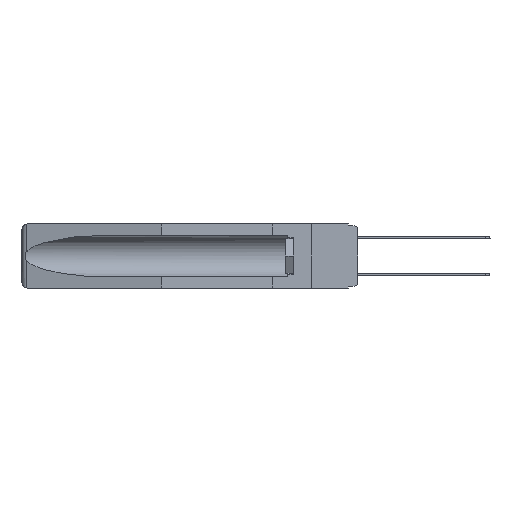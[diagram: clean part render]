
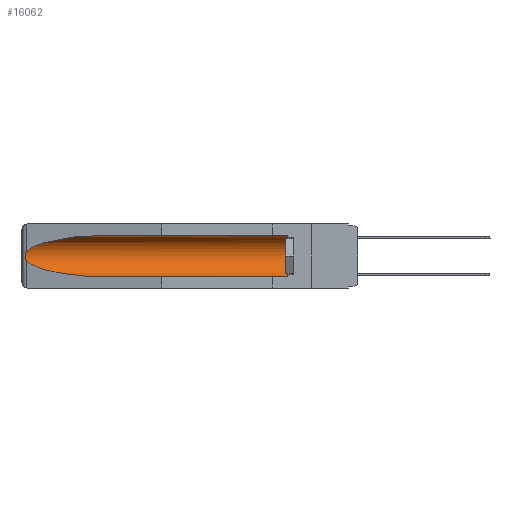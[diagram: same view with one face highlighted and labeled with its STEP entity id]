
A CAD part, left-side view. The second image highlights one B-rep face of the part: STEP entity #16062.
In plain terms, the highlighted cylindrical face has radius 2.857 mm (diameter 5.715 mm), a partial arc.
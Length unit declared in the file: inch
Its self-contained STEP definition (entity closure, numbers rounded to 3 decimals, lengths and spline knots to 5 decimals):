
#847 = CARTESIAN_POINT ( 'NONE',  ( 0.26537, 1.52718, -0.19328 ) ) ;
#1790 = EDGE_LOOP ( 'NONE', ( #23302, #11024, #22615, #20411, #14266, #4914 ) ) ;
#2506 = DIRECTION ( 'NONE',  ( 0., -1., 0. ) ) ;
#2961 = CARTESIAN_POINT ( 'NONE',  ( 0.26597, 1.5296, -0.19026 ) ) ;
#3761 = VERTEX_POINT ( 'NONE', #15420 ) ;
#3801 = AXIS2_PLACEMENT_3D ( 'NONE', #19124, #2506, #17112 ) ;
#4325 = EDGE_CURVE ( 'NONE', #20828, #23090, #21480, .T. ) ;
#4765 = CARTESIAN_POINT ( 'NONE',  ( 0.155, -0.30754, -0.059 ) ) ;
#4914 = ORIENTED_EDGE ( 'NONE', *, *, #7390, .T. ) ;
#5278 = CARTESIAN_POINT ( 'NONE',  ( 0.155, -0.30754, -0.284 ) ) ;
#5702 = EDGE_CURVE ( 'NONE', #15886, #20014, #6276, .T. ) ;
#6276 = B_SPLINE_CURVE_WITH_KNOTS ( 'NONE', 3,
 ( #13979, #10248, #6678, #15747, #21318, #15583, #19163, #23008, #2961, #847 ),
 .UNSPECIFIED., .F., .F.,
 ( 4, 2, 2, 2, 4 ),
 ( 0., 0.00029, 0.00058, 0.00087, 0.00117 ),
 .UNSPECIFIED. ) ;
#6293 = CARTESIAN_POINT ( 'NONE',  ( 0.25451, 1.48313, -0.24835 ) ) ;
#6678 = CARTESIAN_POINT ( 'NONE',  ( 0.26654, 1.53092, -0.15636 ) ) ;
#6847 = CARTESIAN_POINT ( 'NONE',  ( 0.155, 0.126, -0.059 ) ) ;
#7017 = CARTESIAN_POINT ( 'NONE',  ( 0.155, -0.30754, -0.1715 ) ) ;
#7390 = EDGE_CURVE ( 'NONE', #23090, #17053, #17417, .T. ) ;
#7773 = EDGE_CURVE ( 'NONE', #17053, #15886, #18972, .T. ) ;
#7809 = CYLINDRICAL_SURFACE ( 'NONE', #11198, 0.1125 ) ;
#8003 = CARTESIAN_POINT ( 'NONE',  ( 0.26537, 1.52718, -0.14972 ) ) ;
#8981 = CARTESIAN_POINT ( 'NONE',  ( 0.26537, 1.52718, -0.19328 ) ) ;
#9555 = CARTESIAN_POINT ( 'NONE',  ( 0.155, 1.07973, -0.059 ) ) ;
#10248 = CARTESIAN_POINT ( 'NONE',  ( 0.26597, 1.52961, -0.15275 ) ) ;
#11024 = ORIENTED_EDGE ( 'NONE', *, *, #5702, .T. ) ;
#11198 = AXIS2_PLACEMENT_3D ( 'NONE', #7017, #14158, #19795 ) ;
#11314 = CARTESIAN_POINT ( 'NONE',  ( 0.21114, 1.30732, -0.059 ) ) ;
#11334 = CARTESIAN_POINT ( 'NONE',  ( 0.155, 1.07973, -0.059 ) ) ;
#13169 = VECTOR ( 'NONE', #17492, 39.37008 ) ;
#13376 = CARTESIAN_POINT ( 'NONE',  ( 0.25451, 1.48313, -0.09465 ) ) ;
#13979 = CARTESIAN_POINT ( 'NONE',  ( 0.26537, 1.52718, -0.14972 ) ) ;
#14158 = DIRECTION ( 'NONE',  ( 0., 1., 0. ) ) ;
#14266 = ORIENTED_EDGE ( 'NONE', *, *, #4325, .T. ) ;
#14455 = EDGE_CURVE ( 'NONE', #20014, #3761, #14747, .T. ) ;
#14586 = VECTOR ( 'NONE', #19842, 39.37008 ) ;
#14747 =( BOUNDED_CURVE ( )  B_SPLINE_CURVE ( 3, ( #19119, #6293, #21102, #19189 ),
 .UNSPECIFIED., .F., .F. ) 
 B_SPLINE_CURVE_WITH_KNOTS ( ( 4, 4 ),
 ( 0.1948, 1.5708 ),
 .UNSPECIFIED. ) 
 CURVE ( )  GEOMETRIC_REPRESENTATION_ITEM ( )  RATIONAL_B_SPLINE_CURVE ( ( 1., 0.848, 0.848, 1. ) ) 
 REPRESENTATION_ITEM ( '' )  );
#15420 = CARTESIAN_POINT ( 'NONE',  ( 0.155, 1.07973, -0.284 ) ) ;
#15583 = CARTESIAN_POINT ( 'NONE',  ( 0.2675, 1.53308, -0.17534 ) ) ;
#15747 = CARTESIAN_POINT ( 'NONE',  ( 0.2673, 1.5327, -0.16383 ) ) ;
#15886 = VERTEX_POINT ( 'NONE', #19182 ) ;
#16062 = ADVANCED_FACE ( 'NONE', ( #20887 ), #7809, .F. ) ;
#16747 = EDGE_CURVE ( 'NONE', #20828, #3761, #19424, .T. ) ;
#17053 = VERTEX_POINT ( 'NONE', #11334 ) ;
#17112 = DIRECTION ( 'NONE',  ( 0., 0., 1. ) ) ;
#17417 = LINE ( 'NONE', #4765, #13169 ) ;
#17492 = DIRECTION ( 'NONE',  ( 0., 1., 0. ) ) ;
#18972 =( BOUNDED_CURVE ( )  B_SPLINE_CURVE ( 3, ( #9555, #11314, #13376, #8003 ),
 .UNSPECIFIED., .F., .F. ) 
 B_SPLINE_CURVE_WITH_KNOTS ( ( 4, 4 ),
 ( 4.71239, 6.08839 ),
 .UNSPECIFIED. ) 
 CURVE ( )  GEOMETRIC_REPRESENTATION_ITEM ( )  RATIONAL_B_SPLINE_CURVE ( ( 1., 0.848, 0.848, 1. ) ) 
 REPRESENTATION_ITEM ( '' )  );
#19119 = CARTESIAN_POINT ( 'NONE',  ( 0.26537, 1.52718, -0.19328 ) ) ;
#19124 = CARTESIAN_POINT ( 'NONE',  ( 0.155, 0.126, -0.1715 ) ) ;
#19163 = CARTESIAN_POINT ( 'NONE',  ( 0.2673, 1.53269, -0.17917 ) ) ;
#19182 = CARTESIAN_POINT ( 'NONE',  ( 0.26537, 1.52718, -0.14972 ) ) ;
#19189 = CARTESIAN_POINT ( 'NONE',  ( 0.155, 1.07973, -0.284 ) ) ;
#19424 = LINE ( 'NONE', #5278, #14586 ) ;
#19795 = DIRECTION ( 'NONE',  ( 0., 0., 1. ) ) ;
#19842 = DIRECTION ( 'NONE',  ( 0., 1., 0. ) ) ;
#20014 = VERTEX_POINT ( 'NONE', #8981 ) ;
#20411 = ORIENTED_EDGE ( 'NONE', *, *, #16747, .F. ) ;
#20828 = VERTEX_POINT ( 'NONE', #22252 ) ;
#20887 = FACE_OUTER_BOUND ( 'NONE', #1790, .T. ) ;
#21102 = CARTESIAN_POINT ( 'NONE',  ( 0.21114, 1.30732, -0.284 ) ) ;
#21318 = CARTESIAN_POINT ( 'NONE',  ( 0.2675, 1.53308, -0.16763 ) ) ;
#21480 = CIRCLE ( 'NONE', #3801, 0.1125 ) ;
#22252 = CARTESIAN_POINT ( 'NONE',  ( 0.155, 0.126, -0.284 ) ) ;
#22615 = ORIENTED_EDGE ( 'NONE', *, *, #14455, .T. ) ;
#23008 = CARTESIAN_POINT ( 'NONE',  ( 0.26655, 1.53094, -0.18657 ) ) ;
#23090 = VERTEX_POINT ( 'NONE', #6847 ) ;
#23302 = ORIENTED_EDGE ( 'NONE', *, *, #7773, .T. ) ;
